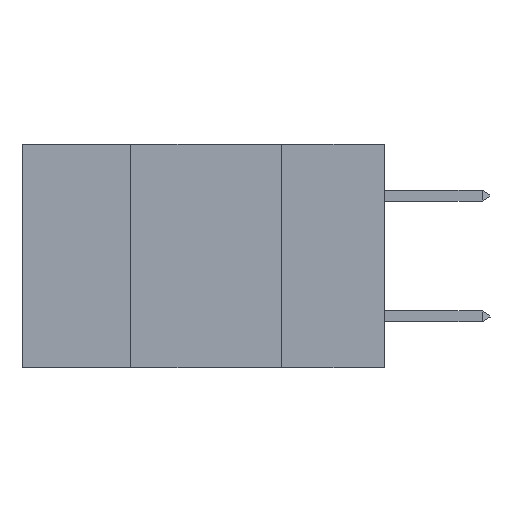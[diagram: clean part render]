
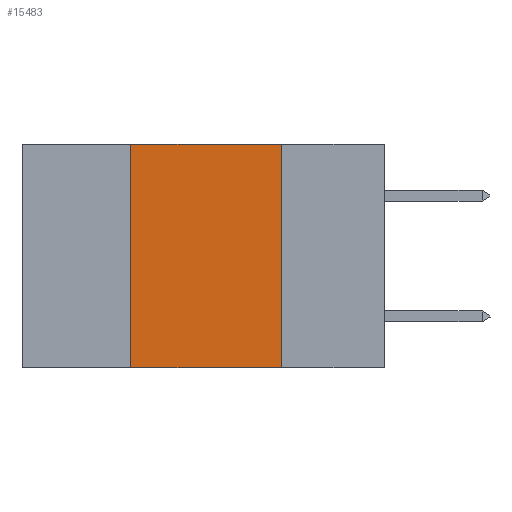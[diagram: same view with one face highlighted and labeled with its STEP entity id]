
A CAD part, left-side view. The second image highlights one B-rep face of the part: STEP entity #15483.
In plain terms, the highlighted planar face has unit normal (-1, 0, 0).
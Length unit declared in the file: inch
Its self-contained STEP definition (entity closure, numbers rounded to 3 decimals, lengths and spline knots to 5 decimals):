
#849 = VERTEX_POINT ( 'NONE', #2176 ) ;
#1476 = CARTESIAN_POINT ( 'NONE',  ( 0., 0.42, 0. ) ) ;
#1761 = VECTOR ( 'NONE', #5238, 39.37008 ) ;
#1896 = LINE ( 'NONE', #9119, #11788 ) ;
#2176 = CARTESIAN_POINT ( 'NONE',  ( 0., 0.42, -0.37 ) ) ;
#2964 = CARTESIAN_POINT ( 'NONE',  ( 0., 0.42, 0. ) ) ;
#3390 = DIRECTION ( 'NONE',  ( 1., 0., 0. ) ) ;
#3451 = VECTOR ( 'NONE', #17024, 39.37008 ) ;
#4153 = EDGE_CURVE ( 'NONE', #19366, #10978, #8763, .T. ) ;
#4672 = CARTESIAN_POINT ( 'NONE',  ( 0., 0.6, 0. ) ) ;
#5238 = DIRECTION ( 'NONE',  ( 0., -1., 0. ) ) ;
#5310 = DIRECTION ( 'NONE',  ( 0., -1., 0. ) ) ;
#5911 = EDGE_CURVE ( 'NONE', #849, #5963, #21963, .T. ) ;
#5963 = VERTEX_POINT ( 'NONE', #1476 ) ;
#6220 = ORIENTED_EDGE ( 'NONE', *, *, #4153, .F. ) ;
#6478 = CARTESIAN_POINT ( 'NONE',  ( 0., 0.17, -0.37 ) ) ;
#7157 = EDGE_LOOP ( 'NONE', ( #6220, #16904, #7711, #16714 ) ) ;
#7711 = ORIENTED_EDGE ( 'NONE', *, *, #5911, .F. ) ;
#8352 = CARTESIAN_POINT ( 'NONE',  ( 0., 0.17, 0. ) ) ;
#8763 = LINE ( 'NONE', #17220, #17647 ) ;
#9119 = CARTESIAN_POINT ( 'NONE',  ( 0., 0.6, -0.37 ) ) ;
#10263 = DIRECTION ( 'NONE',  ( 0., 0., -1. ) ) ;
#10760 = LINE ( 'NONE', #20928, #1761 ) ;
#10978 = VERTEX_POINT ( 'NONE', #6478 ) ;
#11788 = VECTOR ( 'NONE', #5310, 39.37008 ) ;
#12084 = EDGE_CURVE ( 'NONE', #5963, #19366, #10760, .T. ) ;
#13601 = DIRECTION ( 'NONE',  ( 0., 0., -1. ) ) ;
#15188 = PLANE ( 'NONE',  #18605 ) ;
#15483 = ADVANCED_FACE ( 'NONE', ( #17122 ), #15188, .F. ) ;
#16714 = ORIENTED_EDGE ( 'NONE', *, *, #19958, .T. ) ;
#16904 = ORIENTED_EDGE ( 'NONE', *, *, #12084, .F. ) ;
#17024 = DIRECTION ( 'NONE',  ( 0., 0., 1. ) ) ;
#17122 = FACE_OUTER_BOUND ( 'NONE', #7157, .T. ) ;
#17220 = CARTESIAN_POINT ( 'NONE',  ( 0., 0.17, 0. ) ) ;
#17647 = VECTOR ( 'NONE', #10263, 39.37008 ) ;
#18605 = AXIS2_PLACEMENT_3D ( 'NONE', #4672, #3390, #13601 ) ;
#19366 = VERTEX_POINT ( 'NONE', #8352 ) ;
#19958 = EDGE_CURVE ( 'NONE', #849, #10978, #1896, .T. ) ;
#20928 = CARTESIAN_POINT ( 'NONE',  ( 0., 0.6, 0. ) ) ;
#21963 = LINE ( 'NONE', #2964, #3451 ) ;
